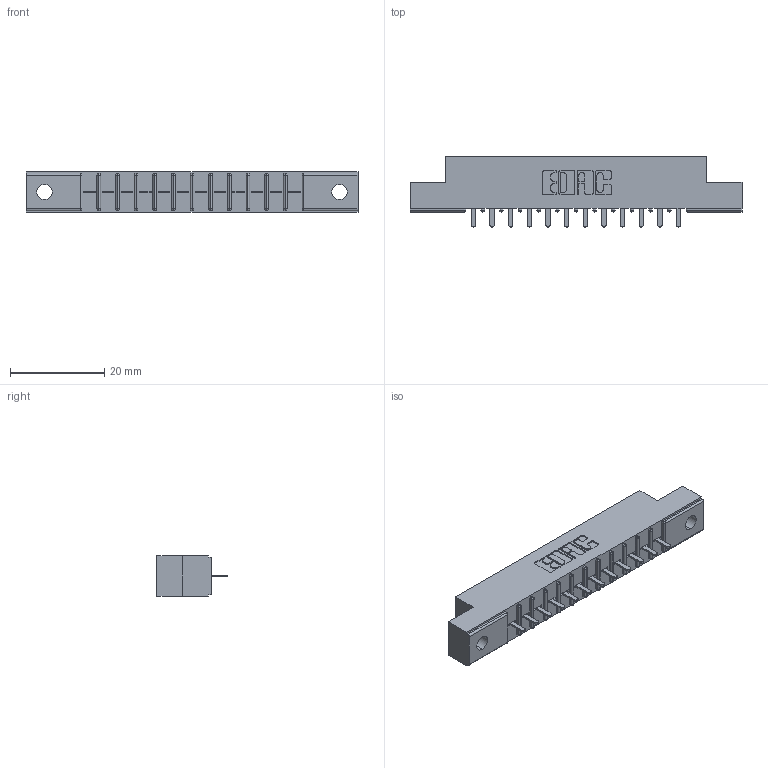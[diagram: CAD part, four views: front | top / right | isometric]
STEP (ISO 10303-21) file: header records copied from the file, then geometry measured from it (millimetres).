
FILE_DESCRIPTION (( 'STEP AP203' ), '1' );
FILE_NAME ('316-012-521-102.STEP', '2018-07-31T00:27:00', ( '' ), ( '' ), 'SwSTEP 2.0', 'SolidWorks 2016', '' );
FILE_SCHEMA (( 'CONFIG_CONTROL_DESIGN' ));
Length unit declared in the file: inch
Products named in the file (3): 306 Part_.128 Dia; 306-290-001_121; 316-012-521-102
Assembly tree (13 placements, depth 2):
  316-012-521-102
    306 Part_.128 Dia
    306-290-001_121  x12
Bounding box: 70.56 x 14.88 x 8.71 mm (x, y, z)
Volume: 4733.6 mm3; surface area: 6329.5 mm2
Topology: 13 solids, 13 shells, 956 faces, 2680 edges, 1720 vertices
Faces by surface type: plane 632, cylinder 276, sphere 48
Entity records: 15035 total; most frequent: CARTESIAN_POINT 2519, ORIENTED_EDGE 2492, DIRECTION 2488, EDGE_CURVE 1246, VECTOR 958, LINE 958, VERTEX_POINT 796, AXIS2_PLACEMENT_3D 765
